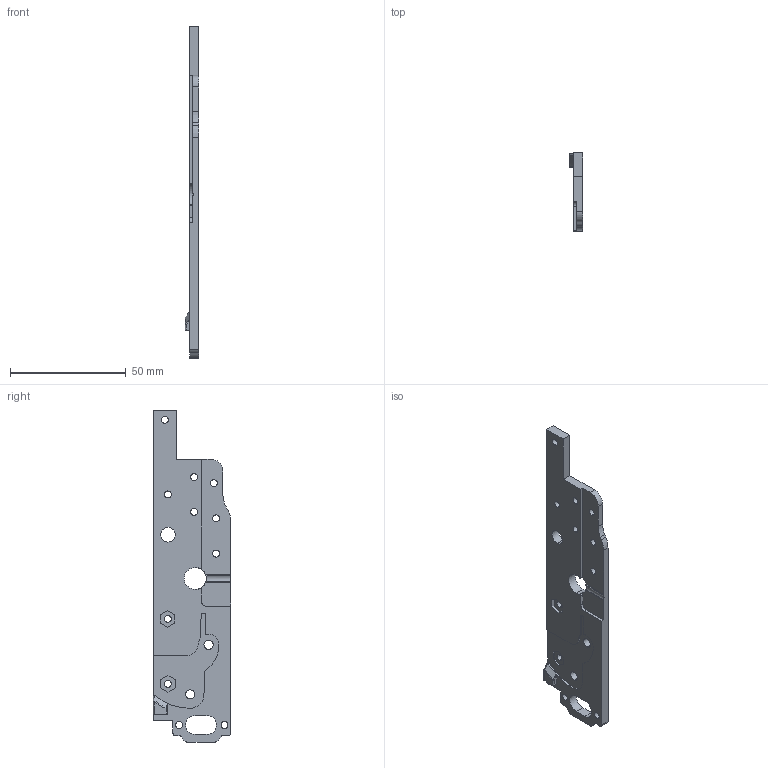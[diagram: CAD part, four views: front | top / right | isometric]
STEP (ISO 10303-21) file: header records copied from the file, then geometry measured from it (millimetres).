
FILE_DESCRIPTION (( 'STEP AP214' ), '1' );
FILE_NAME ('Thunderbolt_Side_Right.STEP', '2021-09-21T22:23:07', ( '' ), ( '' ), 'SwSTEP 2.0', 'SolidWorks 2020', '' );
FILE_SCHEMA (( 'AUTOMOTIVE_DESIGN' ));
Length unit declared in the file: millimetre
Products named in the file (1): Thunderbolt_Side_Right
Bounding box: 6 x 33.43 x 143.21 mm (x, y, z)
Volume: 13905.2 mm3; surface area: 9896.3 mm2
Topology: 1 solids, 1 shells, 115 faces, 330 edges, 216 vertices
Faces by surface type: cylinder 65, plane 43, sphere 3, bspline 2, cone 1, torus 1
Entity records: 3975 total; most frequent: CARTESIAN_POINT 778, DIRECTION 678, ORIENTED_EDGE 656, EDGE_CURVE 328, AXIS2_PLACEMENT_3D 249, VERTEX_POINT 216, LINE 180, VECTOR 180
